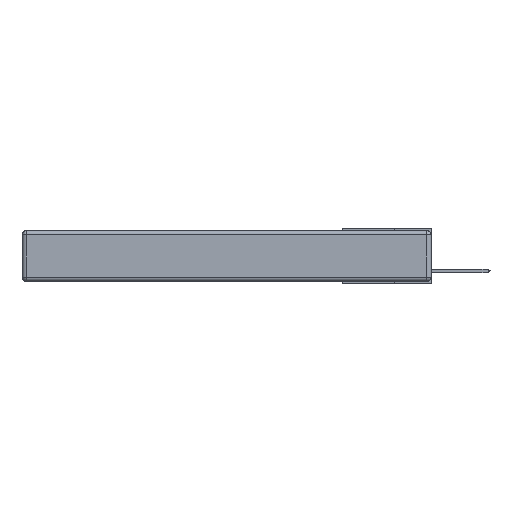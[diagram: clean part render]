
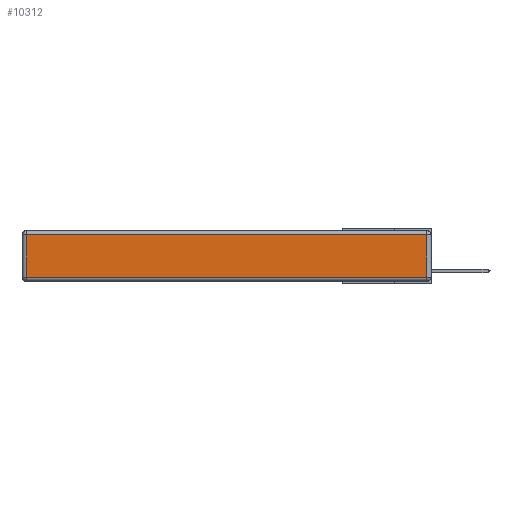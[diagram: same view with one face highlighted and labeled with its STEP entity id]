
A CAD part, left-side view. The second image highlights one B-rep face of the part: STEP entity #10312.
In plain terms, the highlighted planar face has unit normal (-1, 0, 0).
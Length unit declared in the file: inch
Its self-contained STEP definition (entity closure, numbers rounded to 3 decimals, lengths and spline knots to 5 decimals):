
#999 = LINE ( 'NONE', #25977, #17933 ) ;
#2080 = VECTOR ( 'NONE', #25279, 39.37008 ) ;
#2697 = CARTESIAN_POINT ( 'NONE',  ( 0., 2.72, -0.03 ) ) ;
#2818 = DIRECTION ( 'NONE',  ( 0., 0., 1. ) ) ;
#2990 = CARTESIAN_POINT ( 'NONE',  ( 0., 2.72, -0.343 ) ) ;
#3038 = CARTESIAN_POINT ( 'NONE',  ( 0., 0.03, -0.03 ) ) ;
#7466 = VERTEX_POINT ( 'NONE', #9438 ) ;
#8740 = CARTESIAN_POINT ( 'NONE',  ( 0., 0.03, -0.343 ) ) ;
#9438 = CARTESIAN_POINT ( 'NONE',  ( 0., 0.03, -0.313 ) ) ;
#9492 = EDGE_CURVE ( 'NONE', #11500, #20318, #25528, .T. ) ;
#9570 = DIRECTION ( 'NONE',  ( 0., 0., 1. ) ) ;
#9809 = AXIS2_PLACEMENT_3D ( 'NONE', #23704, #23528, #9570 ) ;
#10312 = ADVANCED_FACE ( 'NONE', ( #17965 ), #17537, .T. ) ;
#10526 = LINE ( 'NONE', #2990, #2080 ) ;
#11500 = VERTEX_POINT ( 'NONE', #3038 ) ;
#13484 = DIRECTION ( 'NONE',  ( 0., -1., 0. ) ) ;
#13670 = ORIENTED_EDGE ( 'NONE', *, *, #20155, .T. ) ;
#15011 = DIRECTION ( 'NONE',  ( 0., 1., 0. ) ) ;
#16855 = CARTESIAN_POINT ( 'NONE',  ( 0., 2.75, -0.03 ) ) ;
#16995 = EDGE_CURVE ( 'NONE', #7466, #11500, #24955, .T. ) ;
#17537 = PLANE ( 'NONE',  #9809 ) ;
#17933 = VECTOR ( 'NONE', #13484, 39.37008 ) ;
#17965 = FACE_OUTER_BOUND ( 'NONE', #18641, .T. ) ;
#18589 = VECTOR ( 'NONE', #15011, 39.37008 ) ;
#18641 = EDGE_LOOP ( 'NONE', ( #13670, #19444, #23208, #20293 ) ) ;
#19444 = ORIENTED_EDGE ( 'NONE', *, *, #16995, .T. ) ;
#20155 = EDGE_CURVE ( 'NONE', #23781, #7466, #999, .T. ) ;
#20293 = ORIENTED_EDGE ( 'NONE', *, *, #25230, .T. ) ;
#20318 = VERTEX_POINT ( 'NONE', #2697 ) ;
#20955 = CARTESIAN_POINT ( 'NONE',  ( 0., 2.72, -0.313 ) ) ;
#21783 = VECTOR ( 'NONE', #2818, 39.37008 ) ;
#23208 = ORIENTED_EDGE ( 'NONE', *, *, #9492, .T. ) ;
#23528 = DIRECTION ( 'NONE',  ( -1., 0., 0. ) ) ;
#23704 = CARTESIAN_POINT ( 'NONE',  ( 0., 0., -0.343 ) ) ;
#23781 = VERTEX_POINT ( 'NONE', #20955 ) ;
#24955 = LINE ( 'NONE', #8740, #21783 ) ;
#25230 = EDGE_CURVE ( 'NONE', #20318, #23781, #10526, .T. ) ;
#25279 = DIRECTION ( 'NONE',  ( 0., 0., -1. ) ) ;
#25528 = LINE ( 'NONE', #16855, #18589 ) ;
#25977 = CARTESIAN_POINT ( 'NONE',  ( 0., 0., -0.313 ) ) ;
